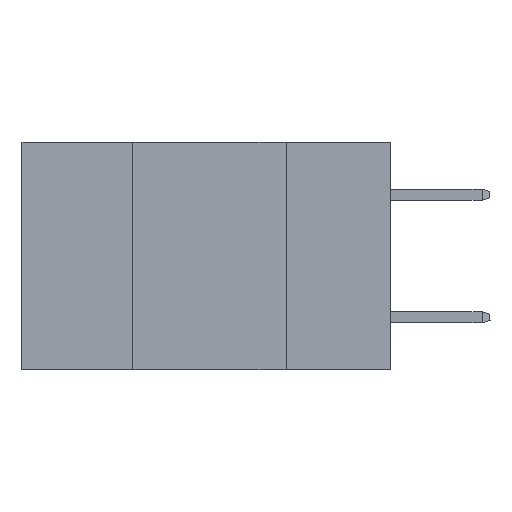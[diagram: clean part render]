
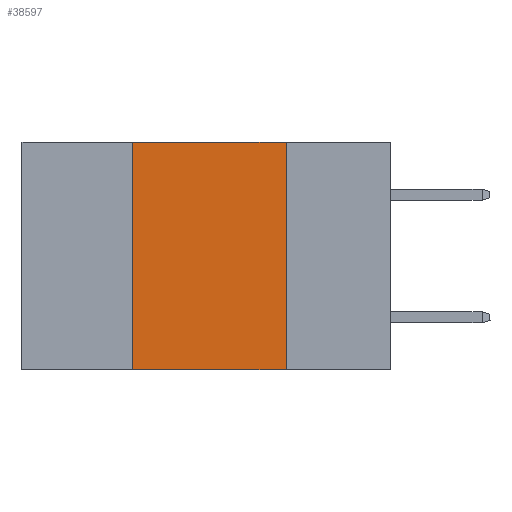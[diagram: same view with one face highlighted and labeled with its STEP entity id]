
A CAD part, left-side view. The second image highlights one B-rep face of the part: STEP entity #38597.
In plain terms, the highlighted planar face has unit normal (-1, 0, 0).
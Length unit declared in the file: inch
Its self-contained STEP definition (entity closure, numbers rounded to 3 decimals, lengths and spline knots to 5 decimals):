
#275 = EDGE_CURVE ( 'NONE', #11767, #42195, #16870, .T. ) ;
#592 = FACE_OUTER_BOUND ( 'NONE', #21322, .T. ) ;
#2204 = CARTESIAN_POINT ( 'NONE',  ( 0., 0.17, 0. ) ) ;
#4264 = PLANE ( 'NONE',  #5759 ) ;
#4339 = EDGE_CURVE ( 'NONE', #42195, #21908, #29147, .T. ) ;
#5618 = VECTOR ( 'NONE', #25266, 39.37008 ) ;
#5759 = AXIS2_PLACEMENT_3D ( 'NONE', #14579, #39797, #35443 ) ;
#6625 = EDGE_CURVE ( 'NONE', #24576, #11767, #35473, .T. ) ;
#7045 = CARTESIAN_POINT ( 'NONE',  ( 0., 0.42, 0. ) ) ;
#7417 = ORIENTED_EDGE ( 'NONE', *, *, #33684, .T. ) ;
#11767 = VERTEX_POINT ( 'NONE', #19701 ) ;
#13764 = CARTESIAN_POINT ( 'NONE',  ( 0., 0.17, -0.37 ) ) ;
#14105 = DIRECTION ( 'NONE',  ( 0., -1., 0. ) ) ;
#14423 = DIRECTION ( 'NONE',  ( 0., -1., 0. ) ) ;
#14579 = CARTESIAN_POINT ( 'NONE',  ( 0., 0.6, 0. ) ) ;
#14707 = CARTESIAN_POINT ( 'NONE',  ( 0., 0.42, -0.37 ) ) ;
#16870 = LINE ( 'NONE', #45092, #19784 ) ;
#18810 = ORIENTED_EDGE ( 'NONE', *, *, #6625, .F. ) ;
#19701 = CARTESIAN_POINT ( 'NONE',  ( 0., 0.42, 0. ) ) ;
#19784 = VECTOR ( 'NONE', #14105, 39.37008 ) ;
#21288 = ORIENTED_EDGE ( 'NONE', *, *, #4339, .F. ) ;
#21322 = EDGE_LOOP ( 'NONE', ( #21288, #42004, #18810, #7417 ) ) ;
#21908 = VERTEX_POINT ( 'NONE', #13764 ) ;
#24576 = VERTEX_POINT ( 'NONE', #14707 ) ;
#25266 = DIRECTION ( 'NONE',  ( 0., 0., -1. ) ) ;
#28997 = VECTOR ( 'NONE', #14423, 39.37008 ) ;
#29147 = LINE ( 'NONE', #31706, #5618 ) ;
#29669 = DIRECTION ( 'NONE',  ( 0., 0., 1. ) ) ;
#31706 = CARTESIAN_POINT ( 'NONE',  ( 0., 0.17, 0. ) ) ;
#33684 = EDGE_CURVE ( 'NONE', #24576, #21908, #42419, .T. ) ;
#35443 = DIRECTION ( 'NONE',  ( 0., 0., -1. ) ) ;
#35473 = LINE ( 'NONE', #7045, #36625 ) ;
#36625 = VECTOR ( 'NONE', #29669, 39.37008 ) ;
#38597 = ADVANCED_FACE ( 'NONE', ( #592 ), #4264, .F. ) ;
#39797 = DIRECTION ( 'NONE',  ( 1., 0., 0. ) ) ;
#41967 = CARTESIAN_POINT ( 'NONE',  ( 0., 0.6, -0.37 ) ) ;
#42004 = ORIENTED_EDGE ( 'NONE', *, *, #275, .F. ) ;
#42195 = VERTEX_POINT ( 'NONE', #2204 ) ;
#42419 = LINE ( 'NONE', #41967, #28997 ) ;
#45092 = CARTESIAN_POINT ( 'NONE',  ( 0., 0.6, 0. ) ) ;
